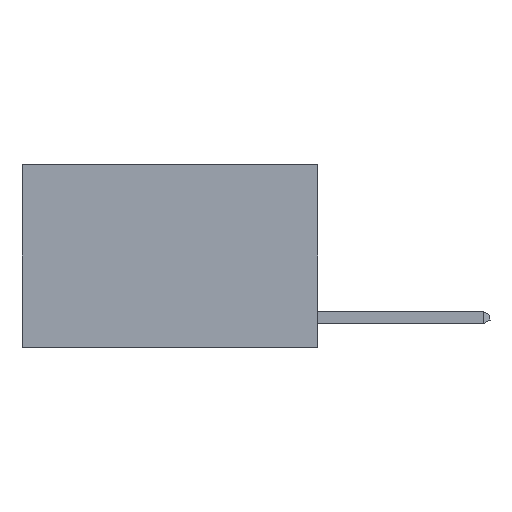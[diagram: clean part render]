
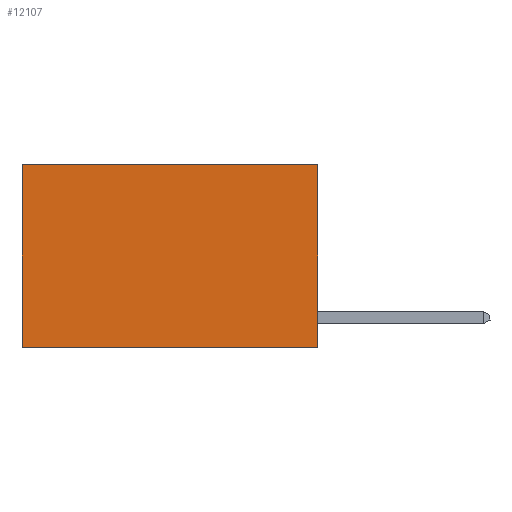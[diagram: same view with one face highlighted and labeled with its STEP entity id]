
A CAD part, left-side view. The second image highlights one B-rep face of the part: STEP entity #12107.
In plain terms, the highlighted planar face has unit normal (-1, 0, 0).
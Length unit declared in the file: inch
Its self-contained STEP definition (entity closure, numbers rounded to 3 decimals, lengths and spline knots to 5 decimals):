
#1293 = VERTEX_POINT ( 'NONE', #14000 ) ;
#1377 = CARTESIAN_POINT ( 'NONE',  ( 0.2625, 0., 0. ) ) ;
#2451 = AXIS2_PLACEMENT_3D ( 'NONE', #17396, #19067, #9237 ) ;
#2539 = VERTEX_POINT ( 'NONE', #4158 ) ;
#4158 = CARTESIAN_POINT ( 'NONE',  ( 0.2625, 0.6, -0.37 ) ) ;
#4227 = CARTESIAN_POINT ( 'NONE',  ( 0.2625, 0., -0.37 ) ) ;
#4297 = VECTOR ( 'NONE', #18554, 39.37008 ) ;
#5147 = FACE_OUTER_BOUND ( 'NONE', #16850, .T. ) ;
#5468 = CARTESIAN_POINT ( 'NONE',  ( 0.2625, 0.6, 0. ) ) ;
#5883 = DIRECTION ( 'NONE',  ( 0., 1., 0. ) ) ;
#6128 = VECTOR ( 'NONE', #7569, 39.37008 ) ;
#6784 = EDGE_CURVE ( 'NONE', #1293, #2539, #19033, .T. ) ;
#7569 = DIRECTION ( 'NONE',  ( 0., 0., -1. ) ) ;
#8816 = VERTEX_POINT ( 'NONE', #18809 ) ;
#9237 = DIRECTION ( 'NONE',  ( 0., 0., -1. ) ) ;
#9239 = ORIENTED_EDGE ( 'NONE', *, *, #13331, .F. ) ;
#9246 = VERTEX_POINT ( 'NONE', #21404 ) ;
#10564 = LINE ( 'NONE', #19096, #6128 ) ;
#12107 = ADVANCED_FACE ( 'NONE', ( #5147 ), #20633, .F. ) ;
#12695 = ORIENTED_EDGE ( 'NONE', *, *, #20241, .T. ) ;
#13331 = EDGE_CURVE ( 'NONE', #9246, #1293, #10564, .T. ) ;
#14000 = CARTESIAN_POINT ( 'NONE',  ( 0.2625, 0., -0.37 ) ) ;
#15930 = VECTOR ( 'NONE', #19543, 39.37008 ) ;
#16656 = EDGE_CURVE ( 'NONE', #8816, #2539, #16924, .T. ) ;
#16850 = EDGE_LOOP ( 'NONE', ( #21257, #20455, #9239, #12695 ) ) ;
#16924 = LINE ( 'NONE', #5468, #4297 ) ;
#16952 = LINE ( 'NONE', #1377, #15930 ) ;
#17396 = CARTESIAN_POINT ( 'NONE',  ( 0.2625, 0., 0. ) ) ;
#18519 = VECTOR ( 'NONE', #5883, 39.37008 ) ;
#18554 = DIRECTION ( 'NONE',  ( 0., 0., -1. ) ) ;
#18809 = CARTESIAN_POINT ( 'NONE',  ( 0.2625, 0.6, 0. ) ) ;
#19033 = LINE ( 'NONE', #4227, #18519 ) ;
#19067 = DIRECTION ( 'NONE',  ( 1., 0., 0. ) ) ;
#19096 = CARTESIAN_POINT ( 'NONE',  ( 0.2625, 0., 0. ) ) ;
#19543 = DIRECTION ( 'NONE',  ( 0., 1., 0. ) ) ;
#20241 = EDGE_CURVE ( 'NONE', #9246, #8816, #16952, .T. ) ;
#20455 = ORIENTED_EDGE ( 'NONE', *, *, #6784, .F. ) ;
#20633 = PLANE ( 'NONE',  #2451 ) ;
#21257 = ORIENTED_EDGE ( 'NONE', *, *, #16656, .T. ) ;
#21404 = CARTESIAN_POINT ( 'NONE',  ( 0.2625, 0., 0. ) ) ;
